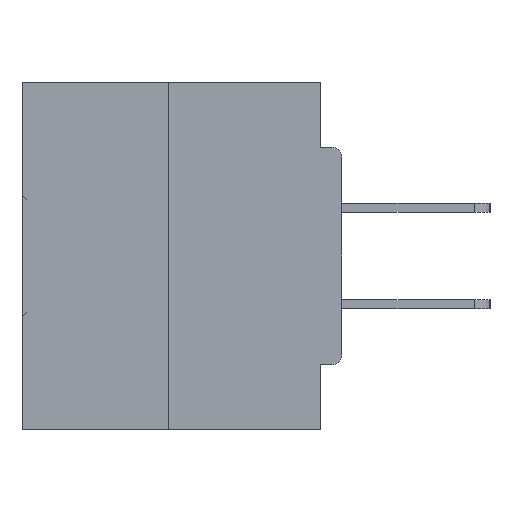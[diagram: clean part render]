
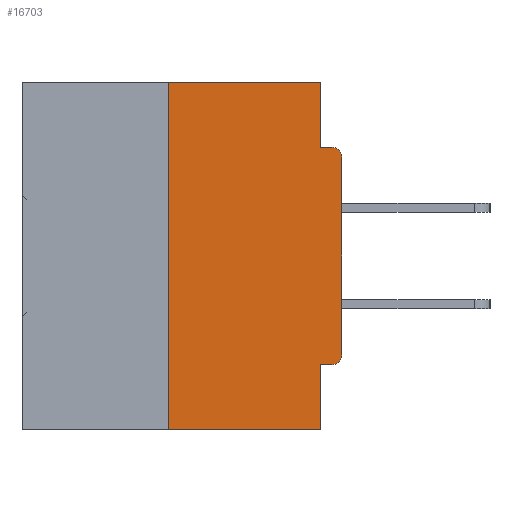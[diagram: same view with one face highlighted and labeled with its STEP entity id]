
A CAD part, left-side view. The second image highlights one B-rep face of the part: STEP entity #16703.
In plain terms, the highlighted planar face has unit normal (-1, 0, 0).
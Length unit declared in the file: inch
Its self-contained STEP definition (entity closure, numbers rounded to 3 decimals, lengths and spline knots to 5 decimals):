
#265 = VERTEX_POINT ( 'NONE', #19378 ) ;
#2494 = CARTESIAN_POINT ( 'NONE',  ( 0., 0.031, -0.5 ) ) ;
#2755 = CARTESIAN_POINT ( 'NONE',  ( 0., 0.25, 0. ) ) ;
#3036 = LINE ( 'NONE', #42372, #16744 ) ;
#4430 = EDGE_CURVE ( 'NONE', #33399, #14830, #8148, .T. ) ;
#4539 = EDGE_CURVE ( 'NONE', #14830, #38726, #44480, .T. ) ;
#6795 = CARTESIAN_POINT ( 'NONE',  ( 0., 0., 0. ) ) ;
#7820 = CARTESIAN_POINT ( 'NONE',  ( 0., 0., -0.1085 ) ) ;
#8148 = CIRCLE ( 'NONE', #18880, 0.015 ) ;
#9449 = VERTEX_POINT ( 'NONE', #40143 ) ;
#9738 = EDGE_CURVE ( 'NONE', #265, #27763, #12864, .T. ) ;
#9850 = CARTESIAN_POINT ( 'NONE',  ( 0., 0., -0.0935 ) ) ;
#10015 = DIRECTION ( 'NONE',  ( -1., 0., 0. ) ) ;
#10159 = DIRECTION ( 'NONE',  ( 0., 0., -1. ) ) ;
#10458 = DIRECTION ( 'NONE',  ( 0., -1., 0. ) ) ;
#11748 = DIRECTION ( 'NONE',  ( 0., 0., 1. ) ) ;
#12385 = DIRECTION ( 'NONE',  ( 0., 1., 0. ) ) ;
#12453 = VECTOR ( 'NONE', #18943, 39.37008 ) ;
#12547 = EDGE_CURVE ( 'NONE', #20000, #21490, #34370, .T. ) ;
#12864 = LINE ( 'NONE', #21037, #42632 ) ;
#12961 = ORIENTED_EDGE ( 'NONE', *, *, #40782, .F. ) ;
#13394 = DIRECTION ( 'NONE',  ( 0., 0., -1. ) ) ;
#13873 = CARTESIAN_POINT ( 'NONE',  ( 0., 0.46, 0. ) ) ;
#13905 = ORIENTED_EDGE ( 'NONE', *, *, #4430, .T. ) ;
#14188 = LINE ( 'NONE', #9850, #24653 ) ;
#14830 = VERTEX_POINT ( 'NONE', #18772 ) ;
#16480 = EDGE_CURVE ( 'NONE', #35559, #27763, #40153, .T. ) ;
#16697 = VECTOR ( 'NONE', #38872, 39.37008 ) ;
#16703 = ADVANCED_FACE ( 'NONE', ( #28554 ), #37949, .F. ) ;
#16744 = VECTOR ( 'NONE', #21461, 39.37008 ) ;
#17078 = CARTESIAN_POINT ( 'NONE',  ( 0., 0.015, -0.1085 ) ) ;
#17520 = CIRCLE ( 'NONE', #42144, 0.015 ) ;
#18184 = ORIENTED_EDGE ( 'NONE', *, *, #19629, .F. ) ;
#18280 = ORIENTED_EDGE ( 'NONE', *, *, #4539, .T. ) ;
#18772 = CARTESIAN_POINT ( 'NONE',  ( 0., 0., -0.3915 ) ) ;
#18880 = AXIS2_PLACEMENT_3D ( 'NONE', #44620, #23654, #41480 ) ;
#18943 = DIRECTION ( 'NONE',  ( 0., 0., 1. ) ) ;
#19378 = CARTESIAN_POINT ( 'NONE',  ( 0., 0.25, -0.5 ) ) ;
#19629 = EDGE_CURVE ( 'NONE', #265, #20000, #21874, .T. ) ;
#20000 = VERTEX_POINT ( 'NONE', #2755 ) ;
#20336 = CARTESIAN_POINT ( 'NONE',  ( 0., 0.46, 0. ) ) ;
#20876 = EDGE_CURVE ( 'NONE', #33399, #35559, #36128, .T. ) ;
#21037 = CARTESIAN_POINT ( 'NONE',  ( 0., 0.46, -0.5 ) ) ;
#21461 = DIRECTION ( 'NONE',  ( 0., 0., -1. ) ) ;
#21490 = VERTEX_POINT ( 'NONE', #35085 ) ;
#21874 = LINE ( 'NONE', #32730, #33987 ) ;
#21928 = VECTOR ( 'NONE', #25428, 39.37008 ) ;
#23654 = DIRECTION ( 'NONE',  ( -1., 0., 0. ) ) ;
#24653 = VECTOR ( 'NONE', #10458, 39.37008 ) ;
#24697 = CARTESIAN_POINT ( 'NONE',  ( 0., 0.031, -0.4065 ) ) ;
#25428 = DIRECTION ( 'NONE',  ( 0., 0., -1. ) ) ;
#25683 = ORIENTED_EDGE ( 'NONE', *, *, #12547, .F. ) ;
#26933 = ORIENTED_EDGE ( 'NONE', *, *, #44900, .F. ) ;
#27763 = VERTEX_POINT ( 'NONE', #2494 ) ;
#27925 = CARTESIAN_POINT ( 'NONE',  ( 0., 0.031, -0.0935 ) ) ;
#28554 = FACE_OUTER_BOUND ( 'NONE', #40212, .T. ) ;
#29236 = ORIENTED_EDGE ( 'NONE', *, *, #9738, .T. ) ;
#29550 = CARTESIAN_POINT ( 'NONE',  ( 0., 0., -0.4065 ) ) ;
#30660 = EDGE_CURVE ( 'NONE', #38726, #9449, #17520, .T. ) ;
#32730 = CARTESIAN_POINT ( 'NONE',  ( 0., 0.25, 0. ) ) ;
#33399 = VERTEX_POINT ( 'NONE', #40182 ) ;
#33987 = VECTOR ( 'NONE', #11748, 39.37008 ) ;
#34370 = LINE ( 'NONE', #13873, #16697 ) ;
#35085 = CARTESIAN_POINT ( 'NONE',  ( 0., 0.031, 0. ) ) ;
#35559 = VERTEX_POINT ( 'NONE', #24697 ) ;
#36128 = LINE ( 'NONE', #29550, #39400 ) ;
#37651 = ORIENTED_EDGE ( 'NONE', *, *, #16480, .F. ) ;
#37949 = PLANE ( 'NONE',  #41029 ) ;
#38726 = VERTEX_POINT ( 'NONE', #7820 ) ;
#38775 = DIRECTION ( 'NONE',  ( 0., -1., 0. ) ) ;
#38872 = DIRECTION ( 'NONE',  ( 0., -1., 0. ) ) ;
#39400 = VECTOR ( 'NONE', #12385, 39.37008 ) ;
#39500 = CARTESIAN_POINT ( 'NONE',  ( 0., 0.031, -0.5 ) ) ;
#40143 = CARTESIAN_POINT ( 'NONE',  ( 0., 0.015, -0.0935 ) ) ;
#40153 = LINE ( 'NONE', #39500, #21928 ) ;
#40182 = CARTESIAN_POINT ( 'NONE',  ( 0., 0.015, -0.4065 ) ) ;
#40212 = EDGE_LOOP ( 'NONE', ( #25683, #18184, #29236, #37651, #44733, #13905, #18280, #45148, #26933, #12961 ) ) ;
#40740 = VERTEX_POINT ( 'NONE', #27925 ) ;
#40782 = EDGE_CURVE ( 'NONE', #21490, #40740, #3036, .T. ) ;
#41029 = AXIS2_PLACEMENT_3D ( 'NONE', #20336, #41733, #13394 ) ;
#41480 = DIRECTION ( 'NONE',  ( 0., 0., -1. ) ) ;
#41733 = DIRECTION ( 'NONE',  ( 1., 0., 0. ) ) ;
#42144 = AXIS2_PLACEMENT_3D ( 'NONE', #17078, #10015, #10159 ) ;
#42372 = CARTESIAN_POINT ( 'NONE',  ( 0., 0.031, 0. ) ) ;
#42632 = VECTOR ( 'NONE', #38775, 39.37008 ) ;
#44480 = LINE ( 'NONE', #6795, #12453 ) ;
#44620 = CARTESIAN_POINT ( 'NONE',  ( 0., 0.015, -0.3915 ) ) ;
#44733 = ORIENTED_EDGE ( 'NONE', *, *, #20876, .F. ) ;
#44900 = EDGE_CURVE ( 'NONE', #40740, #9449, #14188, .T. ) ;
#45148 = ORIENTED_EDGE ( 'NONE', *, *, #30660, .T. ) ;
